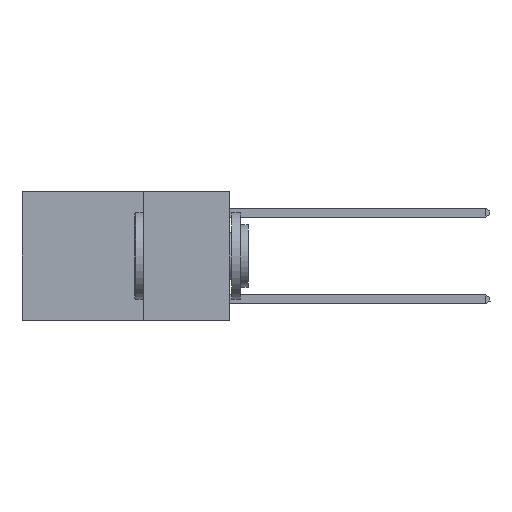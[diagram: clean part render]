
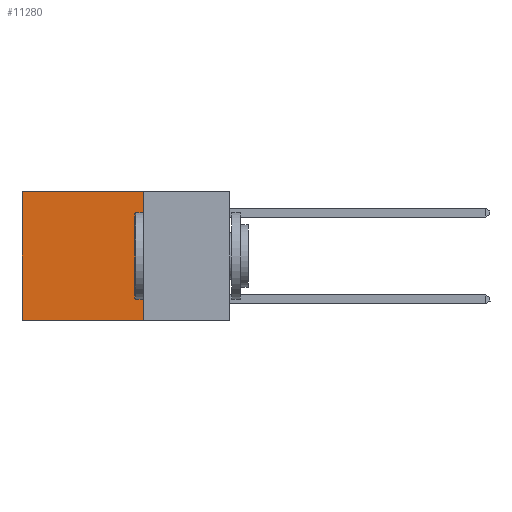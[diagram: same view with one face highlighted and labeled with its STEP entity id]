
A CAD part, left-side view. The second image highlights one B-rep face of the part: STEP entity #11280.
In plain terms, the highlighted planar face has unit normal (-1, 0, 0).
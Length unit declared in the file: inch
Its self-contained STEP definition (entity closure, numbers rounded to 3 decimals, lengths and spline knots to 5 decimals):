
#606 = DIRECTION ( 'NONE',  ( 0., 1., 0. ) ) ;
#1376 = DIRECTION ( 'NONE',  ( 0., 1., 0. ) ) ;
#1685 = CARTESIAN_POINT ( 'NONE',  ( 0.2625, 0.25, 0. ) ) ;
#1817 = CARTESIAN_POINT ( 'NONE',  ( 0.2625, 0.6, -0.37 ) ) ;
#2570 = CARTESIAN_POINT ( 'NONE',  ( 0.2625, 0.25, 0. ) ) ;
#3568 = EDGE_LOOP ( 'NONE', ( #16769, #15216, #16384, #8556 ) ) ;
#3908 = EDGE_CURVE ( 'NONE', #5766, #9419, #9323, .T. ) ;
#3973 = DIRECTION ( 'NONE',  ( 0., 0., -1. ) ) ;
#4645 = VERTEX_POINT ( 'NONE', #8036 ) ;
#5632 = VECTOR ( 'NONE', #606, 39.37008 ) ;
#5766 = VERTEX_POINT ( 'NONE', #1685 ) ;
#7199 = VECTOR ( 'NONE', #15912, 39.37008 ) ;
#7699 = VERTEX_POINT ( 'NONE', #1817 ) ;
#8036 = CARTESIAN_POINT ( 'NONE',  ( 0.2625, 0.25, -0.37 ) ) ;
#8320 = CARTESIAN_POINT ( 'NONE',  ( 0.2625, 0.25, -0.37 ) ) ;
#8420 = EDGE_CURVE ( 'NONE', #4645, #7699, #18167, .T. ) ;
#8556 = ORIENTED_EDGE ( 'NONE', *, *, #3908, .T. ) ;
#8705 = LINE ( 'NONE', #17642, #12038 ) ;
#8792 = AXIS2_PLACEMENT_3D ( 'NONE', #2570, #12340, #3973 ) ;
#9323 = LINE ( 'NONE', #14661, #5632 ) ;
#9419 = VERTEX_POINT ( 'NONE', #10369 ) ;
#10141 = VECTOR ( 'NONE', #1376, 39.37008 ) ;
#10369 = CARTESIAN_POINT ( 'NONE',  ( 0.2625, 0.6, 0. ) ) ;
#10895 = PLANE ( 'NONE',  #8792 ) ;
#10921 = LINE ( 'NONE', #14464, #7199 ) ;
#11280 = ADVANCED_FACE ( 'NONE', ( #15872 ), #10895, .F. ) ;
#11620 = EDGE_CURVE ( 'NONE', #9419, #7699, #10921, .T. ) ;
#11763 = EDGE_CURVE ( 'NONE', #5766, #4645, #8705, .T. ) ;
#11951 = DIRECTION ( 'NONE',  ( 0., 0., -1. ) ) ;
#12038 = VECTOR ( 'NONE', #11951, 39.37008 ) ;
#12340 = DIRECTION ( 'NONE',  ( 1., 0., 0. ) ) ;
#14464 = CARTESIAN_POINT ( 'NONE',  ( 0.2625, 0.6, 0. ) ) ;
#14661 = CARTESIAN_POINT ( 'NONE',  ( 0.2625, 0.25, 0. ) ) ;
#15216 = ORIENTED_EDGE ( 'NONE', *, *, #8420, .F. ) ;
#15872 = FACE_OUTER_BOUND ( 'NONE', #3568, .T. ) ;
#15912 = DIRECTION ( 'NONE',  ( 0., 0., -1. ) ) ;
#16384 = ORIENTED_EDGE ( 'NONE', *, *, #11763, .F. ) ;
#16769 = ORIENTED_EDGE ( 'NONE', *, *, #11620, .T. ) ;
#17642 = CARTESIAN_POINT ( 'NONE',  ( 0.2625, 0.25, 0. ) ) ;
#18167 = LINE ( 'NONE', #8320, #10141 ) ;
